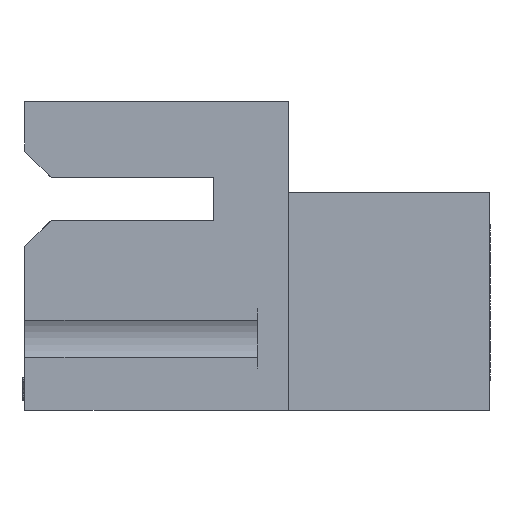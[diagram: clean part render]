
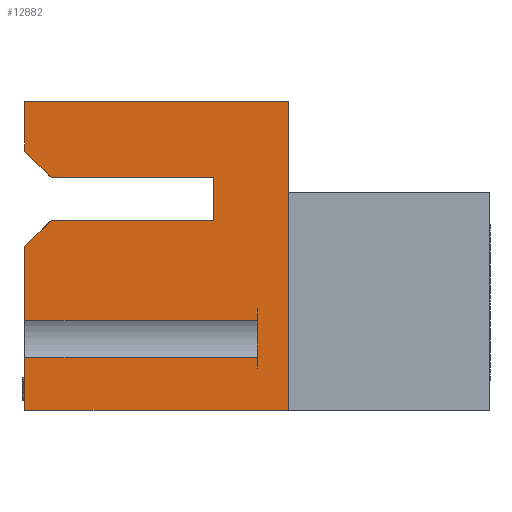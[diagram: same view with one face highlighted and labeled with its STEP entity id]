
A CAD part, left-side view. The second image highlights one B-rep face of the part: STEP entity #12882.
In plain terms, the highlighted planar face has unit normal (-1, 0, 0).
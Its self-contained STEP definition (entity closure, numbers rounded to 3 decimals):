
#8 = CARTESIAN_POINT ( 'NONE',  ( 0., 3.251, -5.182 ) ) ;
#138 = LINE ( 'NONE', #12729, #33572 ) ;
#369 = EDGE_CURVE ( 'NONE', #24194, #24544, #8934, .T. ) ;
#855 = CARTESIAN_POINT ( 'NONE',  ( 0., 1.346, 0. ) ) ;
#917 = LINE ( 'NONE', #12138, #1931 ) ;
#1516 = CARTESIAN_POINT ( 'NONE',  ( 0., 10.363, -3.302 ) ) ;
#1860 = LINE ( 'NONE', #38835, #40361 ) ;
#1931 = VECTOR ( 'NONE', #37910, 1000. ) ;
#2424 = EDGE_CURVE ( 'NONE', #41243, #11304, #1860, .T. ) ;
#3348 = LINE ( 'NONE', #8834, #36773 ) ;
#3554 = EDGE_CURVE ( 'NONE', #25192, #6442, #25378, .T. ) ;
#3817 = VECTOR ( 'NONE', #34076, 1000. ) ;
#4237 = CARTESIAN_POINT ( 'NONE',  ( 0., 11.506, -13.487 ) ) ;
#4393 = VECTOR ( 'NONE', #10771, 1000. ) ;
#4516 = EDGE_CURVE ( 'NONE', #24504, #28255, #9603, .T. ) ;
#5046 = CARTESIAN_POINT ( 'NONE',  ( 0., 0., -5.182 ) ) ;
#5156 = DIRECTION ( 'NONE',  ( 0., 1., 0. ) ) ;
#5388 = FACE_OUTER_BOUND ( 'NONE', #30360, .T. ) ;
#5585 = VERTEX_POINT ( 'NONE', #19038 ) ;
#6179 = VERTEX_POINT ( 'NONE', #29837 ) ;
#6442 = VERTEX_POINT ( 'NONE', #24832 ) ;
#6584 = LINE ( 'NONE', #1516, #33869 ) ;
#7088 = VERTEX_POINT ( 'NONE', #8 ) ;
#7108 = DIRECTION ( 'NONE',  ( 0., -1., 0. ) ) ;
#7329 = ORIENTED_EDGE ( 'NONE', *, *, #9059, .F. ) ;
#7610 = CARTESIAN_POINT ( 'NONE',  ( 0., 11.506, -6.325 ) ) ;
#8569 = EDGE_CURVE ( 'NONE', #5585, #28255, #138, .T. ) ;
#8663 = CARTESIAN_POINT ( 'NONE',  ( 0., 11.506, -2.159 ) ) ;
#8834 = CARTESIAN_POINT ( 'NONE',  ( 0., -8.814, -13.487 ) ) ;
#8934 = LINE ( 'NONE', #23133, #18569 ) ;
#9059 = EDGE_CURVE ( 'NONE', #6442, #24194, #9728, .T. ) ;
#9172 = CARTESIAN_POINT ( 'NONE',  ( 0., 11.506, -9.556 ) ) ;
#9513 = CARTESIAN_POINT ( 'NONE',  ( 0., 3.251, -3.302 ) ) ;
#9603 = LINE ( 'NONE', #36251, #25797 ) ;
#9728 = LINE ( 'NONE', #33143, #34056 ) ;
#10771 = DIRECTION ( 'NONE',  ( 0., 0., 1. ) ) ;
#11302 = EDGE_CURVE ( 'NONE', #25192, #16761, #6584, .T. ) ;
#11304 = VERTEX_POINT ( 'NONE', #17072 ) ;
#11556 = PLANE ( 'NONE',  #23492 ) ;
#12138 = CARTESIAN_POINT ( 'NONE',  ( 0., 3.251, -5.182 ) ) ;
#12729 = CARTESIAN_POINT ( 'NONE',  ( 0., 10.363, -5.182 ) ) ;
#12882 = ADVANCED_FACE ( 'NONE', ( #5388 ), #11556, .F. ) ;
#13235 = CARTESIAN_POINT ( 'NONE',  ( 0., 0., 0. ) ) ;
#13355 = DIRECTION ( 'NONE',  ( 0., 1., 0. ) ) ;
#13404 = CARTESIAN_POINT ( 'NONE',  ( 0., 0., -13.487 ) ) ;
#13799 = DIRECTION ( 'NONE',  ( 0., 0., -1. ) ) ;
#13957 = DIRECTION ( 'NONE',  ( 0., 1., 0. ) ) ;
#14252 = EDGE_CURVE ( 'NONE', #37542, #16761, #17595, .T. ) ;
#14397 = CARTESIAN_POINT ( 'NONE',  ( 0., 1.346, -11.17 ) ) ;
#14526 = CARTESIAN_POINT ( 'NONE',  ( 0., 0., 0. ) ) ;
#14687 = EDGE_CURVE ( 'NONE', #41243, #6179, #22131, .T. ) ;
#15496 = CARTESIAN_POINT ( 'NONE',  ( 0., 11.506, -13.487 ) ) ;
#16761 = VERTEX_POINT ( 'NONE', #18379 ) ;
#17072 = CARTESIAN_POINT ( 'NONE',  ( 0., 11.506, -11.17 ) ) ;
#17595 = LINE ( 'NONE', #33218, #37874 ) ;
#17814 = DIRECTION ( 'NONE',  ( 1., 0., 0. ) ) ;
#17910 = EDGE_CURVE ( 'NONE', #37189, #11304, #18680, .T. ) ;
#17991 = EDGE_CURVE ( 'NONE', #7088, #37542, #917, .T. ) ;
#18221 = DIRECTION ( 'NONE',  ( 0., 0., -1. ) ) ;
#18376 = CARTESIAN_POINT ( 'NONE',  ( 0., 11.506, -13.487 ) ) ;
#18379 = CARTESIAN_POINT ( 'NONE',  ( 0., 10.363, -3.302 ) ) ;
#18569 = VECTOR ( 'NONE', #13799, 1000. ) ;
#18680 = LINE ( 'NONE', #18376, #21169 ) ;
#19038 = CARTESIAN_POINT ( 'NONE',  ( 0., 10.363, -5.182 ) ) ;
#19258 = DIRECTION ( 'NONE',  ( 0., 0.707, -0.707 ) ) ;
#19745 = EDGE_CURVE ( 'NONE', #5585, #7088, #31179, .T. ) ;
#20169 = ORIENTED_EDGE ( 'NONE', *, *, #8569, .T. ) ;
#21169 = VECTOR ( 'NONE', #31245, 1000. ) ;
#21241 = ORIENTED_EDGE ( 'NONE', *, *, #14252, .F. ) ;
#22131 = LINE ( 'NONE', #855, #4393 ) ;
#23133 = CARTESIAN_POINT ( 'NONE',  ( 0., 0., 0. ) ) ;
#23325 = VECTOR ( 'NONE', #30137, 1000. ) ;
#23492 = AXIS2_PLACEMENT_3D ( 'NONE', #14526, #17814, #18221 ) ;
#23995 = DIRECTION ( 'NONE',  ( 0., -0.707, -0.707 ) ) ;
#24194 = VERTEX_POINT ( 'NONE', #13235 ) ;
#24223 = EDGE_CURVE ( 'NONE', #24504, #6179, #41752, .T. ) ;
#24504 = VERTEX_POINT ( 'NONE', #9172 ) ;
#24544 = VERTEX_POINT ( 'NONE', #13404 ) ;
#24832 = CARTESIAN_POINT ( 'NONE',  ( 0., 11.506, 0. ) ) ;
#25192 = VERTEX_POINT ( 'NONE', #8663 ) ;
#25315 = ORIENTED_EDGE ( 'NONE', *, *, #11302, .T. ) ;
#25378 = LINE ( 'NONE', #4237, #23325 ) ;
#25695 = ORIENTED_EDGE ( 'NONE', *, *, #14687, .F. ) ;
#25797 = VECTOR ( 'NONE', #40611, 1000. ) ;
#25947 = ORIENTED_EDGE ( 'NONE', *, *, #4516, .F. ) ;
#27692 = ORIENTED_EDGE ( 'NONE', *, *, #30250, .F. ) ;
#28036 = VECTOR ( 'NONE', #39138, 1000. ) ;
#28255 = VERTEX_POINT ( 'NONE', #7610 ) ;
#29837 = CARTESIAN_POINT ( 'NONE',  ( 0., 1.346, -9.556 ) ) ;
#29946 = ORIENTED_EDGE ( 'NONE', *, *, #369, .F. ) ;
#30135 = ORIENTED_EDGE ( 'NONE', *, *, #2424, .T. ) ;
#30137 = DIRECTION ( 'NONE',  ( 0., 0., 1. ) ) ;
#30250 = EDGE_CURVE ( 'NONE', #24544, #37189, #3348, .T. ) ;
#30360 = EDGE_LOOP ( 'NONE', ( #27692, #29946, #7329, #41812, #25315, #21241, #37833, #30390, #20169, #25947, #39332, #25695, #30135, #35495 ) ) ;
#30390 = ORIENTED_EDGE ( 'NONE', *, *, #19745, .F. ) ;
#31179 = LINE ( 'NONE', #5046, #3817 ) ;
#31245 = DIRECTION ( 'NONE',  ( 0., 0., 1. ) ) ;
#33143 = CARTESIAN_POINT ( 'NONE',  ( 0., 11.506, 0. ) ) ;
#33218 = CARTESIAN_POINT ( 'NONE',  ( 0., 0., -3.302 ) ) ;
#33572 = VECTOR ( 'NONE', #19258, 1000. ) ;
#33869 = VECTOR ( 'NONE', #23995, 1000. ) ;
#34056 = VECTOR ( 'NONE', #7108, 1000. ) ;
#34076 = DIRECTION ( 'NONE',  ( 0., -1., 0. ) ) ;
#35495 = ORIENTED_EDGE ( 'NONE', *, *, #17910, .F. ) ;
#36251 = CARTESIAN_POINT ( 'NONE',  ( 0., 11.506, -13.487 ) ) ;
#36773 = VECTOR ( 'NONE', #5156, 1000. ) ;
#37189 = VERTEX_POINT ( 'NONE', #15496 ) ;
#37542 = VERTEX_POINT ( 'NONE', #9513 ) ;
#37833 = ORIENTED_EDGE ( 'NONE', *, *, #17991, .F. ) ;
#37874 = VECTOR ( 'NONE', #13957, 1000. ) ;
#37910 = DIRECTION ( 'NONE',  ( 0., 0., 1. ) ) ;
#38835 = CARTESIAN_POINT ( 'NONE',  ( 0., 1.346, -11.17 ) ) ;
#38990 = CARTESIAN_POINT ( 'NONE',  ( 0., 1.346, -9.556 ) ) ;
#39138 = DIRECTION ( 'NONE',  ( 0., -1., 0. ) ) ;
#39332 = ORIENTED_EDGE ( 'NONE', *, *, #24223, .T. ) ;
#40361 = VECTOR ( 'NONE', #13355, 1000. ) ;
#40611 = DIRECTION ( 'NONE',  ( 0., 0., 1. ) ) ;
#41243 = VERTEX_POINT ( 'NONE', #14397 ) ;
#41752 = LINE ( 'NONE', #38990, #28036 ) ;
#41812 = ORIENTED_EDGE ( 'NONE', *, *, #3554, .F. ) ;
